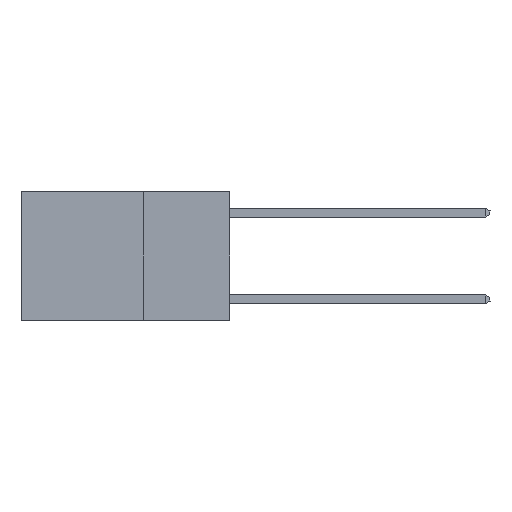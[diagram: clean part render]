
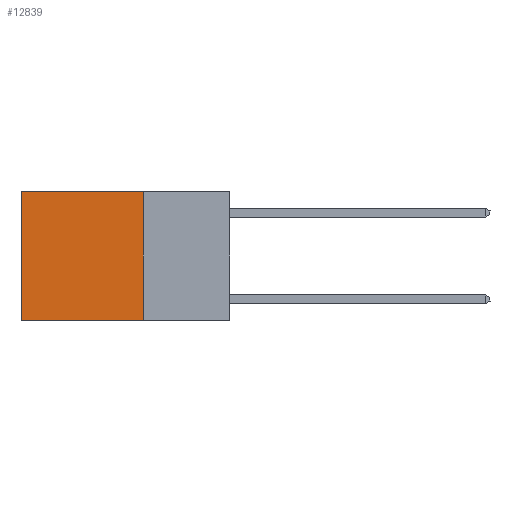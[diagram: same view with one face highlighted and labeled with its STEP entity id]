
A CAD part, left-side view. The second image highlights one B-rep face of the part: STEP entity #12839.
In plain terms, the highlighted planar face has unit normal (-1, 0, 0).
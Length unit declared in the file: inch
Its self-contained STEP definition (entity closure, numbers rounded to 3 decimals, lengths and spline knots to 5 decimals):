
#215 = DIRECTION ( 'NONE',  ( 1., 0., 0. ) ) ;
#361 = PLANE ( 'NONE',  #28076 ) ;
#1968 = VECTOR ( 'NONE', #29529, 39.37008 ) ;
#2281 = LINE ( 'NONE', #23832, #5638 ) ;
#2511 = DIRECTION ( 'NONE',  ( 0., 0., -1. ) ) ;
#4577 = VERTEX_POINT ( 'NONE', #13682 ) ;
#4684 = EDGE_CURVE ( 'NONE', #4577, #21085, #28401, .T. ) ;
#5638 = VECTOR ( 'NONE', #14174, 39.37008 ) ;
#6219 = LINE ( 'NONE', #8225, #17193 ) ;
#7661 = VERTEX_POINT ( 'NONE', #9782 ) ;
#8225 = CARTESIAN_POINT ( 'NONE',  ( 0.2625, 0.25, 0. ) ) ;
#9782 = CARTESIAN_POINT ( 'NONE',  ( 0.2625, 0.25, 0. ) ) ;
#9846 = CARTESIAN_POINT ( 'NONE',  ( 0.2625, 0.6, -0.37 ) ) ;
#9858 = CARTESIAN_POINT ( 'NONE',  ( 0.2625, 0.6, 0. ) ) ;
#10114 = FACE_OUTER_BOUND ( 'NONE', #19749, .T. ) ;
#10249 = EDGE_CURVE ( 'NONE', #7661, #4577, #6219, .T. ) ;
#10532 = CARTESIAN_POINT ( 'NONE',  ( 0.2625, 0.25, -0.37 ) ) ;
#11715 = ORIENTED_EDGE ( 'NONE', *, *, #10249, .T. ) ;
#12839 = ADVANCED_FACE ( 'NONE', ( #10114 ), #361, .F. ) ;
#13682 = CARTESIAN_POINT ( 'NONE',  ( 0.2625, 0.6, 0. ) ) ;
#13699 = EDGE_CURVE ( 'NONE', #7661, #16971, #2281, .T. ) ;
#14174 = DIRECTION ( 'NONE',  ( 0., 0., -1. ) ) ;
#14975 = ORIENTED_EDGE ( 'NONE', *, *, #25050, .F. ) ;
#15370 = DIRECTION ( 'NONE',  ( 0., 1., 0. ) ) ;
#16607 = VECTOR ( 'NONE', #23648, 39.37008 ) ;
#16971 = VERTEX_POINT ( 'NONE', #21162 ) ;
#17193 = VECTOR ( 'NONE', #15370, 39.37008 ) ;
#17420 = ORIENTED_EDGE ( 'NONE', *, *, #4684, .T. ) ;
#19749 = EDGE_LOOP ( 'NONE', ( #17420, #14975, #25282, #11715 ) ) ;
#21085 = VERTEX_POINT ( 'NONE', #9846 ) ;
#21162 = CARTESIAN_POINT ( 'NONE',  ( 0.2625, 0.25, -0.37 ) ) ;
#21301 = CARTESIAN_POINT ( 'NONE',  ( 0.2625, 0.25, 0. ) ) ;
#23648 = DIRECTION ( 'NONE',  ( 0., 0., -1. ) ) ;
#23832 = CARTESIAN_POINT ( 'NONE',  ( 0.2625, 0.25, 0. ) ) ;
#25050 = EDGE_CURVE ( 'NONE', #16971, #21085, #27396, .T. ) ;
#25282 = ORIENTED_EDGE ( 'NONE', *, *, #13699, .F. ) ;
#27396 = LINE ( 'NONE', #10532, #1968 ) ;
#28076 = AXIS2_PLACEMENT_3D ( 'NONE', #21301, #215, #2511 ) ;
#28401 = LINE ( 'NONE', #9858, #16607 ) ;
#29529 = DIRECTION ( 'NONE',  ( 0., 1., 0. ) ) ;
